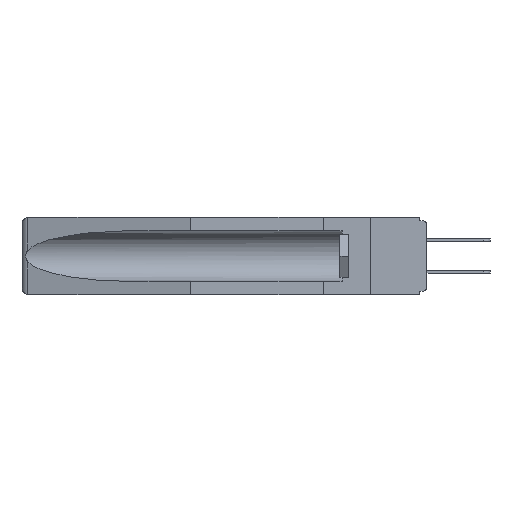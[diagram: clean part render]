
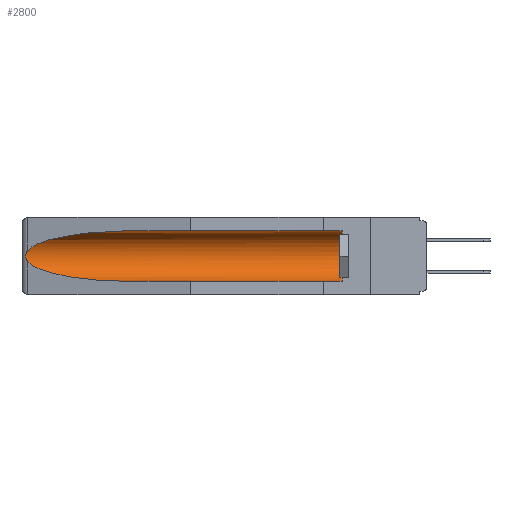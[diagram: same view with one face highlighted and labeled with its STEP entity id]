
A CAD part, left-side view. The second image highlights one B-rep face of the part: STEP entity #2800.
In plain terms, the highlighted cylindrical face has radius 2.857 mm (diameter 5.715 mm), a partial arc.
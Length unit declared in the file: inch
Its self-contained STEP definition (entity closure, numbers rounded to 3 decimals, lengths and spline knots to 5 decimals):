
#447 = AXIS2_PLACEMENT_3D ( 'NONE', #13393, #25444, #15417 ) ;
#2035 = EDGE_CURVE ( 'NONE', #16307, #25858, #16992, .T. ) ;
#2072 = EDGE_CURVE ( 'NONE', #18933, #16307, #23252, .T. ) ;
#2326 = DIRECTION ( 'NONE',  ( 0., 0., 1. ) ) ;
#2608 = CARTESIAN_POINT ( 'NONE',  ( 0.155, 1.07973, -0.059 ) ) ;
#2800 = ADVANCED_FACE ( 'NONE', ( #6683 ), #3237, .F. ) ;
#2995 = CARTESIAN_POINT ( 'NONE',  ( 0.155, 1.07973, -0.059 ) ) ;
#3237 = CYLINDRICAL_SURFACE ( 'NONE', #447, 0.1125 ) ;
#3755 =( BOUNDED_CURVE ( )  B_SPLINE_CURVE ( 3, ( #16626, #10401, #12434, #12686 ),
 .UNSPECIFIED., .F., .F. ) 
 B_SPLINE_CURVE_WITH_KNOTS ( ( 4, 4 ),
 ( 0.1948, 1.5708 ),
 .UNSPECIFIED. ) 
 CURVE ( )  GEOMETRIC_REPRESENTATION_ITEM ( )  RATIONAL_B_SPLINE_CURVE ( ( 1., 0.848, 0.848, 1. ) ) 
 REPRESENTATION_ITEM ( '' )  );
#5157 = CARTESIAN_POINT ( 'NONE',  ( 0.26654, 1.53092, -0.15636 ) ) ;
#5454 = VECTOR ( 'NONE', #20833, 39.37008 ) ;
#5518 = VERTEX_POINT ( 'NONE', #7910 ) ;
#5742 = EDGE_CURVE ( 'NONE', #25858, #24781, #10289, .T. ) ;
#6035 = CARTESIAN_POINT ( 'NONE',  ( 0.155, -0.30754, -0.284 ) ) ;
#6578 = CARTESIAN_POINT ( 'NONE',  ( 0.26655, 1.53094, -0.18657 ) ) ;
#6683 = FACE_OUTER_BOUND ( 'NONE', #13085, .T. ) ;
#6732 = CARTESIAN_POINT ( 'NONE',  ( 0.2673, 1.53269, -0.17917 ) ) ;
#6873 = CARTESIAN_POINT ( 'NONE',  ( 0.155, -0.30754, -0.059 ) ) ;
#7896 = CARTESIAN_POINT ( 'NONE',  ( 0.26597, 1.52961, -0.15275 ) ) ;
#7910 = CARTESIAN_POINT ( 'NONE',  ( 0.155, 1.07973, -0.284 ) ) ;
#8851 = ORIENTED_EDGE ( 'NONE', *, *, #5742, .T. ) ;
#9670 = LINE ( 'NONE', #6035, #18436 ) ;
#10289 =( BOUNDED_CURVE ( )  B_SPLINE_CURVE ( 3, ( #2608, #16561, #16728, #16817 ),
 .UNSPECIFIED., .F., .F. ) 
 B_SPLINE_CURVE_WITH_KNOTS ( ( 4, 4 ),
 ( 4.71239, 6.08839 ),
 .UNSPECIFIED. ) 
 CURVE ( )  GEOMETRIC_REPRESENTATION_ITEM ( )  RATIONAL_B_SPLINE_CURVE ( ( 1., 0.848, 0.848, 1. ) ) 
 REPRESENTATION_ITEM ( '' )  );
#10323 = CARTESIAN_POINT ( 'NONE',  ( 0.155, 0.126, -0.284 ) ) ;
#10401 = CARTESIAN_POINT ( 'NONE',  ( 0.25451, 1.48313, -0.24835 ) ) ;
#11084 = EDGE_CURVE ( 'NONE', #18933, #5518, #9670, .T. ) ;
#12434 = CARTESIAN_POINT ( 'NONE',  ( 0.21114, 1.30732, -0.284 ) ) ;
#12591 = CARTESIAN_POINT ( 'NONE',  ( 0.2675, 1.53308, -0.17534 ) ) ;
#12686 = CARTESIAN_POINT ( 'NONE',  ( 0.155, 1.07973, -0.284 ) ) ;
#13071 = ORIENTED_EDGE ( 'NONE', *, *, #20521, .T. ) ;
#13085 = EDGE_LOOP ( 'NONE', ( #8851, #15235, #13071, #19325, #15352, #17285 ) ) ;
#13165 = CARTESIAN_POINT ( 'NONE',  ( 0.26537, 1.52718, -0.19328 ) ) ;
#13393 = CARTESIAN_POINT ( 'NONE',  ( 0.155, -0.30754, -0.1715 ) ) ;
#14781 = CARTESIAN_POINT ( 'NONE',  ( 0.2673, 1.5327, -0.16383 ) ) ;
#15235 = ORIENTED_EDGE ( 'NONE', *, *, #17221, .T. ) ;
#15352 = ORIENTED_EDGE ( 'NONE', *, *, #2072, .T. ) ;
#15417 = DIRECTION ( 'NONE',  ( 0., 0., 1. ) ) ;
#16097 = DIRECTION ( 'NONE',  ( 0., -1., 0. ) ) ;
#16307 = VERTEX_POINT ( 'NONE', #20080 ) ;
#16561 = CARTESIAN_POINT ( 'NONE',  ( 0.21114, 1.30732, -0.059 ) ) ;
#16626 = CARTESIAN_POINT ( 'NONE',  ( 0.26537, 1.52718, -0.19328 ) ) ;
#16728 = CARTESIAN_POINT ( 'NONE',  ( 0.25451, 1.48313, -0.09465 ) ) ;
#16817 = CARTESIAN_POINT ( 'NONE',  ( 0.26537, 1.52718, -0.14972 ) ) ;
#16992 = LINE ( 'NONE', #6873, #5454 ) ;
#17221 = EDGE_CURVE ( 'NONE', #24781, #21363, #22658, .T. ) ;
#17285 = ORIENTED_EDGE ( 'NONE', *, *, #2035, .T. ) ;
#17748 = CARTESIAN_POINT ( 'NONE',  ( 0.26537, 1.52718, -0.14972 ) ) ;
#18436 = VECTOR ( 'NONE', #18505, 39.37008 ) ;
#18505 = DIRECTION ( 'NONE',  ( 0., 1., 0. ) ) ;
#18540 = CARTESIAN_POINT ( 'NONE',  ( 0.2675, 1.53308, -0.16763 ) ) ;
#18933 = VERTEX_POINT ( 'NONE', #10323 ) ;
#19325 = ORIENTED_EDGE ( 'NONE', *, *, #11084, .F. ) ;
#19606 = CARTESIAN_POINT ( 'NONE',  ( 0.26537, 1.52718, -0.14972 ) ) ;
#20014 = CARTESIAN_POINT ( 'NONE',  ( 0.155, 0.126, -0.1715 ) ) ;
#20080 = CARTESIAN_POINT ( 'NONE',  ( 0.155, 0.126, -0.059 ) ) ;
#20521 = EDGE_CURVE ( 'NONE', #21363, #5518, #3755, .T. ) ;
#20833 = DIRECTION ( 'NONE',  ( 0., 1., 0. ) ) ;
#21363 = VERTEX_POINT ( 'NONE', #13165 ) ;
#22384 = CARTESIAN_POINT ( 'NONE',  ( 0.26537, 1.52718, -0.19328 ) ) ;
#22421 = AXIS2_PLACEMENT_3D ( 'NONE', #20014, #16097, #2326 ) ;
#22569 = CARTESIAN_POINT ( 'NONE',  ( 0.26597, 1.5296, -0.19026 ) ) ;
#22658 = B_SPLINE_CURVE_WITH_KNOTS ( 'NONE', 3,
 ( #19606, #7896, #5157, #14781, #18540, #12591, #6732, #6578, #22569, #22384 ),
 .UNSPECIFIED., .F., .F.,
 ( 4, 2, 2, 2, 4 ),
 ( 0., 0.00029, 0.00058, 0.00087, 0.00117 ),
 .UNSPECIFIED. ) ;
#23252 = CIRCLE ( 'NONE', #22421, 0.1125 ) ;
#24781 = VERTEX_POINT ( 'NONE', #17748 ) ;
#25444 = DIRECTION ( 'NONE',  ( 0., 1., 0. ) ) ;
#25858 = VERTEX_POINT ( 'NONE', #2995 ) ;
